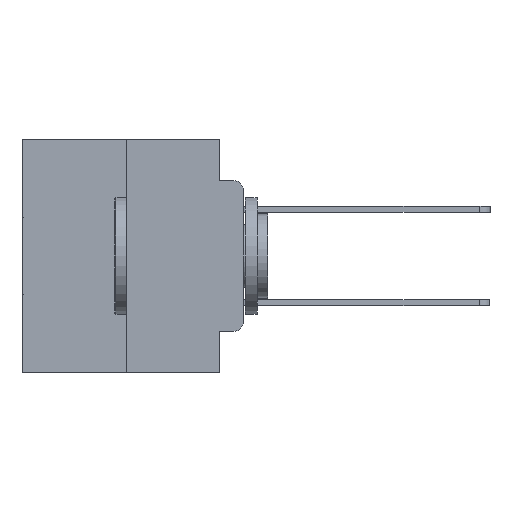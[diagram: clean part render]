
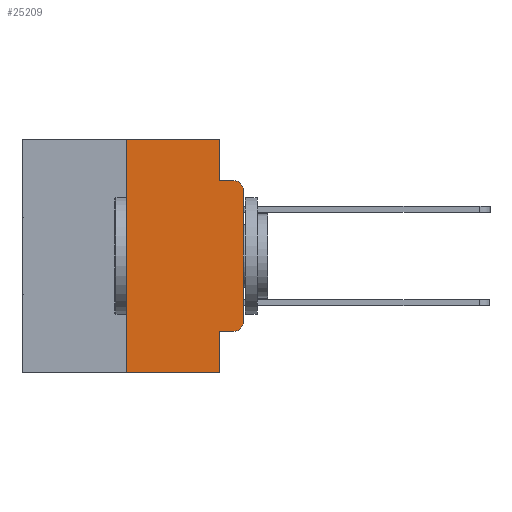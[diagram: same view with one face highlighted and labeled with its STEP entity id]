
A CAD part, left-side view. The second image highlights one B-rep face of the part: STEP entity #25209.
In plain terms, the highlighted planar face has unit normal (-1, 0, 0).
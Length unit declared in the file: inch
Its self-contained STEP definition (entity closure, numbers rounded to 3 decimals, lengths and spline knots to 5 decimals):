
#273 = DIRECTION ( 'NONE',  ( 0., 0., 1. ) ) ;
#503 = LINE ( 'NONE', #29626, #25035 ) ;
#605 = DIRECTION ( 'NONE',  ( -1., 0., 0. ) ) ;
#903 = AXIS2_PLACEMENT_3D ( 'NONE', #14902, #605, #17252 ) ;
#1207 = DIRECTION ( 'NONE',  ( 0., -1., 0. ) ) ;
#1336 = AXIS2_PLACEMENT_3D ( 'NONE', #29971, #29421, #29752 ) ;
#1641 = VECTOR ( 'NONE', #10424, 39.37008 ) ;
#1874 = EDGE_CURVE ( 'NONE', #24747, #16801, #8144, .T. ) ;
#2034 = ORIENTED_EDGE ( 'NONE', *, *, #19528, .T. ) ;
#2222 = ORIENTED_EDGE ( 'NONE', *, *, #29235, .T. ) ;
#2631 = EDGE_CURVE ( 'NONE', #4710, #15002, #13314, .T. ) ;
#2768 = ORIENTED_EDGE ( 'NONE', *, *, #6442, .F. ) ;
#3203 = EDGE_LOOP ( 'NONE', ( #9525, #2034, #2768, #16221, #6532, #27690, #2222, #16414, #5230, #27136 ) ) ;
#4710 = VERTEX_POINT ( 'NONE', #18725 ) ;
#5230 = ORIENTED_EDGE ( 'NONE', *, *, #21188, .T. ) ;
#6442 = EDGE_CURVE ( 'NONE', #22179, #12433, #6501, .T. ) ;
#6501 = LINE ( 'NONE', #27607, #30244 ) ;
#6532 = ORIENTED_EDGE ( 'NONE', *, *, #28502, .F. ) ;
#6904 = DIRECTION ( 'NONE',  ( 0., 0., -1. ) ) ;
#7248 = CARTESIAN_POINT ( 'NONE',  ( 0., 0.051, -0.5 ) ) ;
#8144 = CIRCLE ( 'NONE', #1336, 0.02 ) ;
#8207 = VECTOR ( 'NONE', #6904, 39.37008 ) ;
#9090 = DIRECTION ( 'NONE',  ( 0., 0., -1. ) ) ;
#9430 = VECTOR ( 'NONE', #273, 39.37008 ) ;
#9525 = ORIENTED_EDGE ( 'NONE', *, *, #13822, .T. ) ;
#10053 = FACE_OUTER_BOUND ( 'NONE', #3203, .T. ) ;
#10424 = DIRECTION ( 'NONE',  ( 0., -1., 0. ) ) ;
#12169 = LINE ( 'NONE', #23293, #18400 ) ;
#12186 = CARTESIAN_POINT ( 'NONE',  ( 0., 0.02, -0.4115 ) ) ;
#12433 = VERTEX_POINT ( 'NONE', #18611 ) ;
#13139 = CARTESIAN_POINT ( 'NONE',  ( 0., 0.051, -0.4115 ) ) ;
#13314 = LINE ( 'NONE', #23455, #25150 ) ;
#13394 = CARTESIAN_POINT ( 'NONE',  ( 0., 0., -0.1085 ) ) ;
#13822 = EDGE_CURVE ( 'NONE', #16801, #14169, #15744, .T. ) ;
#14106 = DIRECTION ( 'NONE',  ( 0., 0., -1. ) ) ;
#14169 = VERTEX_POINT ( 'NONE', #13394 ) ;
#14358 = LINE ( 'NONE', #22234, #1641 ) ;
#14902 = CARTESIAN_POINT ( 'NONE',  ( 0., 0.02, -0.1085 ) ) ;
#15002 = VERTEX_POINT ( 'NONE', #30181 ) ;
#15447 = LINE ( 'NONE', #13139, #28027 ) ;
#15450 = DIRECTION ( 'NONE',  ( 0., -1., 0. ) ) ;
#15744 = LINE ( 'NONE', #28722, #9430 ) ;
#16221 = ORIENTED_EDGE ( 'NONE', *, *, #17598, .F. ) ;
#16414 = ORIENTED_EDGE ( 'NONE', *, *, #28111, .F. ) ;
#16503 = CARTESIAN_POINT ( 'NONE',  ( 0., 0.051, 0. ) ) ;
#16801 = VERTEX_POINT ( 'NONE', #20434 ) ;
#17252 = DIRECTION ( 'NONE',  ( 0., 0., -1. ) ) ;
#17576 = VERTEX_POINT ( 'NONE', #18734 ) ;
#17598 = EDGE_CURVE ( 'NONE', #17576, #22179, #25623, .T. ) ;
#17755 = AXIS2_PLACEMENT_3D ( 'NONE', #23544, #28273, #14106 ) ;
#18242 = VERTEX_POINT ( 'NONE', #22105 ) ;
#18400 = VECTOR ( 'NONE', #9090, 39.37008 ) ;
#18611 = CARTESIAN_POINT ( 'NONE',  ( 0., 0.02, -0.0885 ) ) ;
#18725 = CARTESIAN_POINT ( 'NONE',  ( 0., 0.25, -0.5 ) ) ;
#18734 = CARTESIAN_POINT ( 'NONE',  ( 0., 0.051, 0. ) ) ;
#19284 = DIRECTION ( 'NONE',  ( 0., 0., 1. ) ) ;
#19528 = EDGE_CURVE ( 'NONE', #14169, #12433, #22973, .T. ) ;
#20434 = CARTESIAN_POINT ( 'NONE',  ( 0., 0., -0.3915 ) ) ;
#21188 = EDGE_CURVE ( 'NONE', #18242, #24747, #15447, .T. ) ;
#21439 = CARTESIAN_POINT ( 'NONE',  ( 0., 0.051, -0.0885 ) ) ;
#22105 = CARTESIAN_POINT ( 'NONE',  ( 0., 0.051, -0.4115 ) ) ;
#22179 = VERTEX_POINT ( 'NONE', #21439 ) ;
#22234 = CARTESIAN_POINT ( 'NONE',  ( 0., 0.473, 0. ) ) ;
#22973 = CIRCLE ( 'NONE', #903, 0.02 ) ;
#23293 = CARTESIAN_POINT ( 'NONE',  ( 0., 0.051, 0. ) ) ;
#23455 = CARTESIAN_POINT ( 'NONE',  ( 0., 0.25, 0. ) ) ;
#23544 = CARTESIAN_POINT ( 'NONE',  ( 0., 0.473, 0. ) ) ;
#24747 = VERTEX_POINT ( 'NONE', #12186 ) ;
#25035 = VECTOR ( 'NONE', #15450, 39.37008 ) ;
#25150 = VECTOR ( 'NONE', #19284, 39.37008 ) ;
#25209 = ADVANCED_FACE ( 'NONE', ( #10053 ), #25897, .F. ) ;
#25623 = LINE ( 'NONE', #16503, #8207 ) ;
#25897 = PLANE ( 'NONE',  #17755 ) ;
#26926 = VERTEX_POINT ( 'NONE', #7248 ) ;
#27136 = ORIENTED_EDGE ( 'NONE', *, *, #1874, .T. ) ;
#27607 = CARTESIAN_POINT ( 'NONE',  ( 0., 0.051, -0.0885 ) ) ;
#27690 = ORIENTED_EDGE ( 'NONE', *, *, #2631, .F. ) ;
#28027 = VECTOR ( 'NONE', #1207, 39.37008 ) ;
#28111 = EDGE_CURVE ( 'NONE', #18242, #26926, #12169, .T. ) ;
#28273 = DIRECTION ( 'NONE',  ( 1., 0., 0. ) ) ;
#28502 = EDGE_CURVE ( 'NONE', #15002, #17576, #14358, .T. ) ;
#28722 = CARTESIAN_POINT ( 'NONE',  ( 0., 0., 0. ) ) ;
#29235 = EDGE_CURVE ( 'NONE', #4710, #26926, #503, .T. ) ;
#29421 = DIRECTION ( 'NONE',  ( -1., 0., 0. ) ) ;
#29626 = CARTESIAN_POINT ( 'NONE',  ( 0., 0.473, -0.5 ) ) ;
#29752 = DIRECTION ( 'NONE',  ( 0., 0., -1. ) ) ;
#29971 = CARTESIAN_POINT ( 'NONE',  ( 0., 0.02, -0.3915 ) ) ;
#30003 = DIRECTION ( 'NONE',  ( 0., -1., 0. ) ) ;
#30181 = CARTESIAN_POINT ( 'NONE',  ( 0., 0.25, 0. ) ) ;
#30244 = VECTOR ( 'NONE', #30003, 39.37008 ) ;
